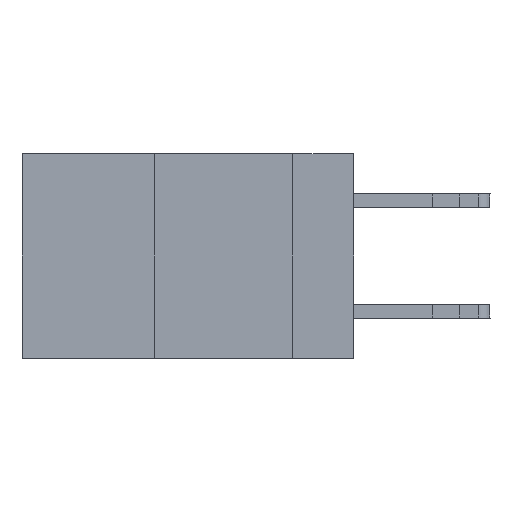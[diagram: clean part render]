
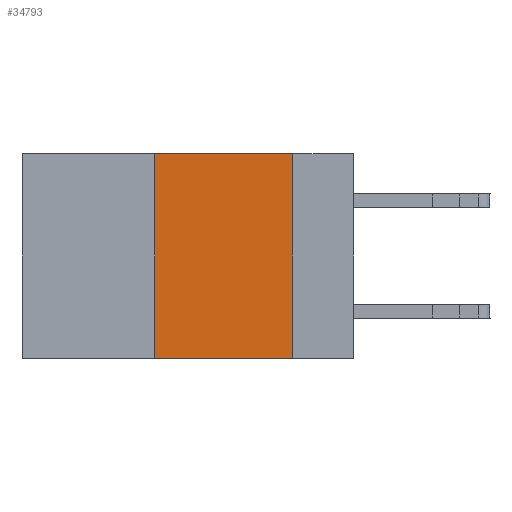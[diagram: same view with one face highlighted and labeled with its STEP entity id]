
A CAD part, left-side view. The second image highlights one B-rep face of the part: STEP entity #34793.
In plain terms, the highlighted planar face has unit normal (-1, 0, 0).
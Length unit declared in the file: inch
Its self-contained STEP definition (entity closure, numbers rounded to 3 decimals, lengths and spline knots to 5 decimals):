
#195 = CARTESIAN_POINT ( 'NONE',  ( 0., 0.36, 0. ) ) ;
#1340 = PLANE ( 'NONE',  #16669 ) ;
#1565 = VERTEX_POINT ( 'NONE', #195 ) ;
#2394 = EDGE_LOOP ( 'NONE', ( #33675, #14355, #31527, #35030 ) ) ;
#5305 = LINE ( 'NONE', #16936, #12777 ) ;
#6276 = CARTESIAN_POINT ( 'NONE',  ( 0., 0.6, 0. ) ) ;
#7777 = DIRECTION ( 'NONE',  ( 0., -1., 0. ) ) ;
#8291 = FACE_OUTER_BOUND ( 'NONE', #2394, .T. ) ;
#9185 = EDGE_CURVE ( 'NONE', #31393, #31877, #5305, .T. ) ;
#9883 = CARTESIAN_POINT ( 'NONE',  ( 0., 0.6, 0. ) ) ;
#11191 = CARTESIAN_POINT ( 'NONE',  ( 0., 0.36, -0.37 ) ) ;
#12709 = DIRECTION ( 'NONE',  ( 1., 0., 0. ) ) ;
#12777 = VECTOR ( 'NONE', #7777, 39.37008 ) ;
#13031 = DIRECTION ( 'NONE',  ( 0., 0., 1. ) ) ;
#13525 = EDGE_CURVE ( 'NONE', #1565, #29210, #31738, .T. ) ;
#14355 = ORIENTED_EDGE ( 'NONE', *, *, #13525, .F. ) ;
#15214 = VECTOR ( 'NONE', #19911, 39.37008 ) ;
#16669 = AXIS2_PLACEMENT_3D ( 'NONE', #9883, #12709, #32226 ) ;
#16936 = CARTESIAN_POINT ( 'NONE',  ( 0., 0.6, -0.37 ) ) ;
#19679 = CARTESIAN_POINT ( 'NONE',  ( 0., 0.11, 0. ) ) ;
#19911 = DIRECTION ( 'NONE',  ( 0., 0., -1. ) ) ;
#20965 = CARTESIAN_POINT ( 'NONE',  ( 0., 0.11, 0. ) ) ;
#26325 = CARTESIAN_POINT ( 'NONE',  ( 0., 0.36, 0. ) ) ;
#27078 = LINE ( 'NONE', #19679, #15214 ) ;
#27602 = CARTESIAN_POINT ( 'NONE',  ( 0., 0.11, -0.37 ) ) ;
#28474 = EDGE_CURVE ( 'NONE', #31393, #1565, #29059, .T. ) ;
#29059 = LINE ( 'NONE', #26325, #35134 ) ;
#29210 = VERTEX_POINT ( 'NONE', #20965 ) ;
#31393 = VERTEX_POINT ( 'NONE', #11191 ) ;
#31416 = EDGE_CURVE ( 'NONE', #29210, #31877, #27078, .T. ) ;
#31527 = ORIENTED_EDGE ( 'NONE', *, *, #28474, .F. ) ;
#31738 = LINE ( 'NONE', #6276, #34772 ) ;
#31877 = VERTEX_POINT ( 'NONE', #27602 ) ;
#32226 = DIRECTION ( 'NONE',  ( 0., 0., -1. ) ) ;
#32551 = DIRECTION ( 'NONE',  ( 0., -1., 0. ) ) ;
#33675 = ORIENTED_EDGE ( 'NONE', *, *, #31416, .F. ) ;
#34772 = VECTOR ( 'NONE', #32551, 39.37008 ) ;
#34793 = ADVANCED_FACE ( 'NONE', ( #8291 ), #1340, .F. ) ;
#35030 = ORIENTED_EDGE ( 'NONE', *, *, #9185, .T. ) ;
#35134 = VECTOR ( 'NONE', #13031, 39.37008 ) ;
